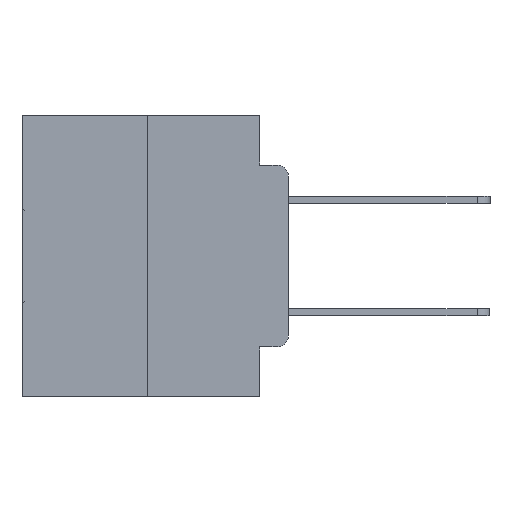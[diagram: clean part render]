
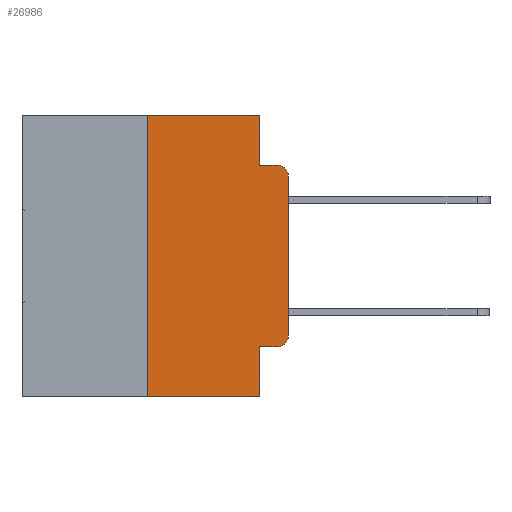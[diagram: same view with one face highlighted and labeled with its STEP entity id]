
A CAD part, left-side view. The second image highlights one B-rep face of the part: STEP entity #26986.
In plain terms, the highlighted planar face has unit normal (-1, 0, 0).
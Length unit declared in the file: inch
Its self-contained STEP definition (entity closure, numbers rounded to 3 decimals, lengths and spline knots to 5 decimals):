
#207 = VERTEX_POINT ( 'NONE', #4772 ) ;
#274 = EDGE_CURVE ( 'NONE', #18612, #207, #3577, .T. ) ;
#452 = CARTESIAN_POINT ( 'NONE',  ( 0., 0.051, 0. ) ) ;
#1444 = ORIENTED_EDGE ( 'NONE', *, *, #31793, .T. ) ;
#1718 = VECTOR ( 'NONE', #11181, 39.37008 ) ;
#2173 = CARTESIAN_POINT ( 'NONE',  ( 0., 0.051, 0. ) ) ;
#2249 = EDGE_CURVE ( 'NONE', #207, #11725, #18689, .T. ) ;
#2542 = EDGE_CURVE ( 'NONE', #30387, #11725, #18284, .T. ) ;
#2833 = ORIENTED_EDGE ( 'NONE', *, *, #31186, .F. ) ;
#3124 = CARTESIAN_POINT ( 'NONE',  ( 0., 0.051, -0.5 ) ) ;
#3135 = DIRECTION ( 'NONE',  ( 0., 0., -1. ) ) ;
#3577 = LINE ( 'NONE', #13655, #14566 ) ;
#3859 = ORIENTED_EDGE ( 'NONE', *, *, #2249, .T. ) ;
#3912 = EDGE_CURVE ( 'NONE', #28740, #28098, #8475, .T. ) ;
#4560 = ORIENTED_EDGE ( 'NONE', *, *, #3912, .F. ) ;
#4772 = CARTESIAN_POINT ( 'NONE',  ( 0., 0., -0.1085 ) ) ;
#6043 = CARTESIAN_POINT ( 'NONE',  ( 0., 0., -0.3915 ) ) ;
#6273 = ORIENTED_EDGE ( 'NONE', *, *, #2542, .F. ) ;
#6382 = DIRECTION ( 'NONE',  ( 0., -1., 0. ) ) ;
#6478 = VECTOR ( 'NONE', #29011, 39.37008 ) ;
#6658 = VECTOR ( 'NONE', #25280, 39.37008 ) ;
#6751 = DIRECTION ( 'NONE',  ( 0., -1., 0. ) ) ;
#8259 = CARTESIAN_POINT ( 'NONE',  ( 0., 0.02, -0.1085 ) ) ;
#8475 = LINE ( 'NONE', #24063, #1718 ) ;
#9318 = EDGE_CURVE ( 'NONE', #28098, #30387, #26987, .T. ) ;
#9348 = AXIS2_PLACEMENT_3D ( 'NONE', #8259, #18107, #3135 ) ;
#9936 = LINE ( 'NONE', #13898, #28606 ) ;
#10096 = DIRECTION ( 'NONE',  ( 0., 0., -1. ) ) ;
#11181 = DIRECTION ( 'NONE',  ( 0., -1., 0. ) ) ;
#11658 = CARTESIAN_POINT ( 'NONE',  ( 0., 0.051, -0.0885 ) ) ;
#11725 = VERTEX_POINT ( 'NONE', #29827 ) ;
#12038 = LINE ( 'NONE', #14268, #25033 ) ;
#12411 = VERTEX_POINT ( 'NONE', #3124 ) ;
#12838 = VECTOR ( 'NONE', #19654, 39.37008 ) ;
#13520 = DIRECTION ( 'NONE',  ( -1., 0., 0. ) ) ;
#13655 = CARTESIAN_POINT ( 'NONE',  ( 0., 0., 0. ) ) ;
#13898 = CARTESIAN_POINT ( 'NONE',  ( 0., 0.473, -0.5 ) ) ;
#14268 = CARTESIAN_POINT ( 'NONE',  ( 0., 0.051, -0.4115 ) ) ;
#14566 = VECTOR ( 'NONE', #17156, 39.37008 ) ;
#15414 = AXIS2_PLACEMENT_3D ( 'NONE', #27076, #24770, #10096 ) ;
#16834 = EDGE_CURVE ( 'NONE', #25482, #12411, #9936, .T. ) ;
#16945 = EDGE_LOOP ( 'NONE', ( #28118, #3859, #6273, #25083, #4560, #2833, #26885, #21668, #1444, #19440 ) ) ;
#17156 = DIRECTION ( 'NONE',  ( 0., 0., 1. ) ) ;
#17514 = VECTOR ( 'NONE', #28967, 39.37008 ) ;
#18107 = DIRECTION ( 'NONE',  ( -1., 0., 0. ) ) ;
#18284 = LINE ( 'NONE', #11658, #17514 ) ;
#18612 = VERTEX_POINT ( 'NONE', #6043 ) ;
#18689 = CIRCLE ( 'NONE', #9348, 0.02 ) ;
#19092 = CARTESIAN_POINT ( 'NONE',  ( 0., 0.25, 0. ) ) ;
#19440 = ORIENTED_EDGE ( 'NONE', *, *, #21432, .T. ) ;
#19543 = CARTESIAN_POINT ( 'NONE',  ( 0., 0.051, 0. ) ) ;
#19654 = DIRECTION ( 'NONE',  ( 0., 0., -1. ) ) ;
#19943 = PLANE ( 'NONE',  #15414 ) ;
#20464 = AXIS2_PLACEMENT_3D ( 'NONE', #28030, #13520, #30487 ) ;
#20921 = CARTESIAN_POINT ( 'NONE',  ( 0., 0.051, -0.0885 ) ) ;
#21219 = VERTEX_POINT ( 'NONE', #29637 ) ;
#21432 = EDGE_CURVE ( 'NONE', #29896, #18612, #31650, .T. ) ;
#21476 = CARTESIAN_POINT ( 'NONE',  ( 0., 0.02, -0.4115 ) ) ;
#21668 = ORIENTED_EDGE ( 'NONE', *, *, #24725, .F. ) ;
#23503 = CARTESIAN_POINT ( 'NONE',  ( 0., 0.25, -0.5 ) ) ;
#24063 = CARTESIAN_POINT ( 'NONE',  ( 0., 0.473, 0. ) ) ;
#24725 = EDGE_CURVE ( 'NONE', #21219, #12411, #31482, .T. ) ;
#24770 = DIRECTION ( 'NONE',  ( 1., 0., 0. ) ) ;
#25033 = VECTOR ( 'NONE', #6751, 39.37008 ) ;
#25083 = ORIENTED_EDGE ( 'NONE', *, *, #9318, .F. ) ;
#25280 = DIRECTION ( 'NONE',  ( 0., 0., -1. ) ) ;
#25482 = VERTEX_POINT ( 'NONE', #23503 ) ;
#26625 = CARTESIAN_POINT ( 'NONE',  ( 0., 0.25, 0. ) ) ;
#26885 = ORIENTED_EDGE ( 'NONE', *, *, #16834, .T. ) ;
#26986 = ADVANCED_FACE ( 'NONE', ( #29666 ), #19943, .F. ) ;
#26987 = LINE ( 'NONE', #452, #6658 ) ;
#27076 = CARTESIAN_POINT ( 'NONE',  ( 0., 0.473, 0. ) ) ;
#28030 = CARTESIAN_POINT ( 'NONE',  ( 0., 0.02, -0.3915 ) ) ;
#28098 = VERTEX_POINT ( 'NONE', #19543 ) ;
#28118 = ORIENTED_EDGE ( 'NONE', *, *, #274, .T. ) ;
#28606 = VECTOR ( 'NONE', #6382, 39.37008 ) ;
#28740 = VERTEX_POINT ( 'NONE', #19092 ) ;
#28967 = DIRECTION ( 'NONE',  ( 0., -1., 0. ) ) ;
#29011 = DIRECTION ( 'NONE',  ( 0., 0., 1. ) ) ;
#29637 = CARTESIAN_POINT ( 'NONE',  ( 0., 0.051, -0.4115 ) ) ;
#29666 = FACE_OUTER_BOUND ( 'NONE', #16945, .T. ) ;
#29827 = CARTESIAN_POINT ( 'NONE',  ( 0., 0.02, -0.0885 ) ) ;
#29896 = VERTEX_POINT ( 'NONE', #21476 ) ;
#30387 = VERTEX_POINT ( 'NONE', #20921 ) ;
#30487 = DIRECTION ( 'NONE',  ( 0., 0., -1. ) ) ;
#31186 = EDGE_CURVE ( 'NONE', #25482, #28740, #31750, .T. ) ;
#31482 = LINE ( 'NONE', #2173, #12838 ) ;
#31650 = CIRCLE ( 'NONE', #20464, 0.02 ) ;
#31750 = LINE ( 'NONE', #26625, #6478 ) ;
#31793 = EDGE_CURVE ( 'NONE', #21219, #29896, #12038, .T. ) ;
